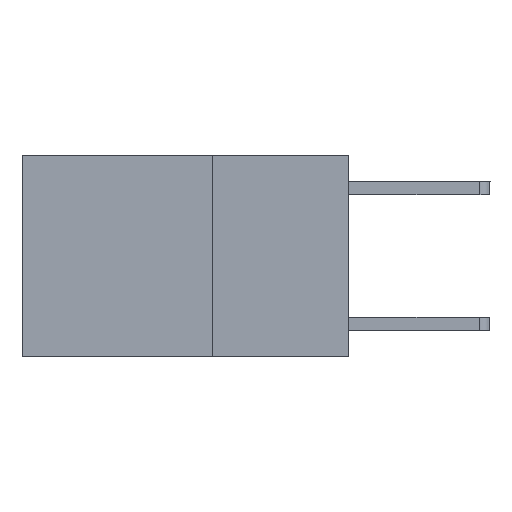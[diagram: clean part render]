
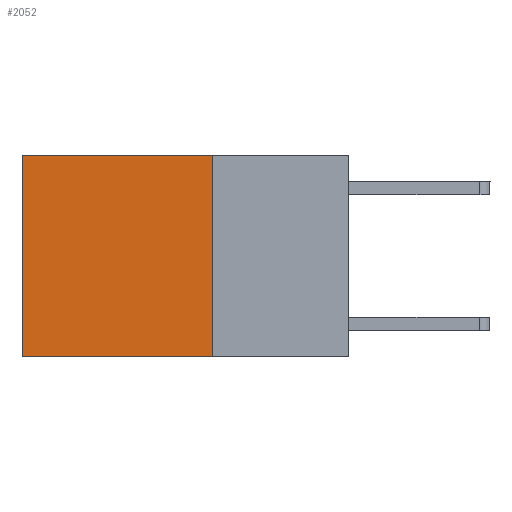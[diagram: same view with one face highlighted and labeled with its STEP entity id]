
A CAD part, left-side view. The second image highlights one B-rep face of the part: STEP entity #2052.
In plain terms, the highlighted planar face has unit normal (-1, 0, 0).
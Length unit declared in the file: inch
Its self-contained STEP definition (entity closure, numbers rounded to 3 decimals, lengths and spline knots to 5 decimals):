
#314 = CARTESIAN_POINT ( 'NONE',  ( 0.2625, 0.25, -0.37 ) ) ;
#1064 = LINE ( 'NONE', #1861, #4181 ) ;
#1619 = EDGE_CURVE ( 'NONE', #4079, #2394, #7381, .T. ) ;
#1854 = CARTESIAN_POINT ( 'NONE',  ( 0.2625, 0.25, 0. ) ) ;
#1861 = CARTESIAN_POINT ( 'NONE',  ( 0.2625, 0.25, -0.37 ) ) ;
#1897 = CARTESIAN_POINT ( 'NONE',  ( 0.2625, 0.6, -0.37 ) ) ;
#2052 = ADVANCED_FACE ( 'NONE', ( #2963 ), #5261, .F. ) ;
#2226 = EDGE_LOOP ( 'NONE', ( #5517, #5065, #6090, #6568 ) ) ;
#2376 = EDGE_CURVE ( 'NONE', #8419, #6818, #1064, .T. ) ;
#2394 = VERTEX_POINT ( 'NONE', #8669 ) ;
#2862 = DIRECTION ( 'NONE',  ( 1., 0., 0. ) ) ;
#2926 = CARTESIAN_POINT ( 'NONE',  ( 0.2625, 0.25, 0. ) ) ;
#2963 = FACE_OUTER_BOUND ( 'NONE', #2226, .T. ) ;
#3017 = DIRECTION ( 'NONE',  ( 0., 1., 0. ) ) ;
#3047 = DIRECTION ( 'NONE',  ( 0., 0., -1. ) ) ;
#3221 = VECTOR ( 'NONE', #5027, 39.37008 ) ;
#4079 = VERTEX_POINT ( 'NONE', #1854 ) ;
#4181 = VECTOR ( 'NONE', #7863, 39.37008 ) ;
#4242 = LINE ( 'NONE', #7987, #3221 ) ;
#5027 = DIRECTION ( 'NONE',  ( 0., 0., -1. ) ) ;
#5065 = ORIENTED_EDGE ( 'NONE', *, *, #2376, .F. ) ;
#5261 = PLANE ( 'NONE',  #6203 ) ;
#5301 = EDGE_CURVE ( 'NONE', #2394, #6818, #4242, .T. ) ;
#5449 = CARTESIAN_POINT ( 'NONE',  ( 0.2625, 0.25, 0. ) ) ;
#5517 = ORIENTED_EDGE ( 'NONE', *, *, #5301, .T. ) ;
#5937 = DIRECTION ( 'NONE',  ( 0., 0., -1. ) ) ;
#6090 = ORIENTED_EDGE ( 'NONE', *, *, #6496, .F. ) ;
#6203 = AXIS2_PLACEMENT_3D ( 'NONE', #6594, #2862, #5937 ) ;
#6496 = EDGE_CURVE ( 'NONE', #4079, #8419, #7521, .T. ) ;
#6568 = ORIENTED_EDGE ( 'NONE', *, *, #1619, .T. ) ;
#6594 = CARTESIAN_POINT ( 'NONE',  ( 0.2625, 0.25, 0. ) ) ;
#6802 = VECTOR ( 'NONE', #3047, 39.37008 ) ;
#6818 = VERTEX_POINT ( 'NONE', #1897 ) ;
#7381 = LINE ( 'NONE', #2926, #8261 ) ;
#7521 = LINE ( 'NONE', #5449, #6802 ) ;
#7863 = DIRECTION ( 'NONE',  ( 0., 1., 0. ) ) ;
#7987 = CARTESIAN_POINT ( 'NONE',  ( 0.2625, 0.6, 0. ) ) ;
#8261 = VECTOR ( 'NONE', #3017, 39.37008 ) ;
#8419 = VERTEX_POINT ( 'NONE', #314 ) ;
#8669 = CARTESIAN_POINT ( 'NONE',  ( 0.2625, 0.6, 0. ) ) ;
